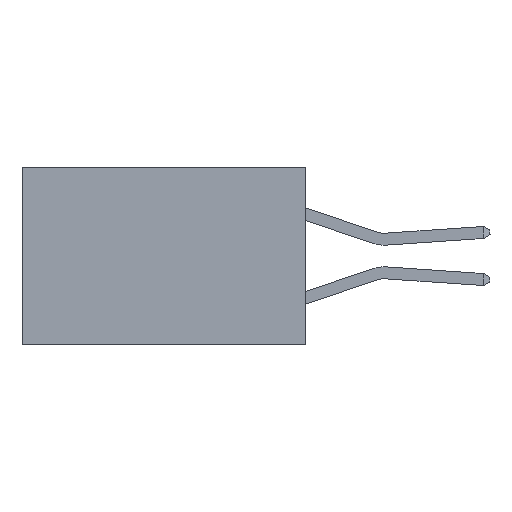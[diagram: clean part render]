
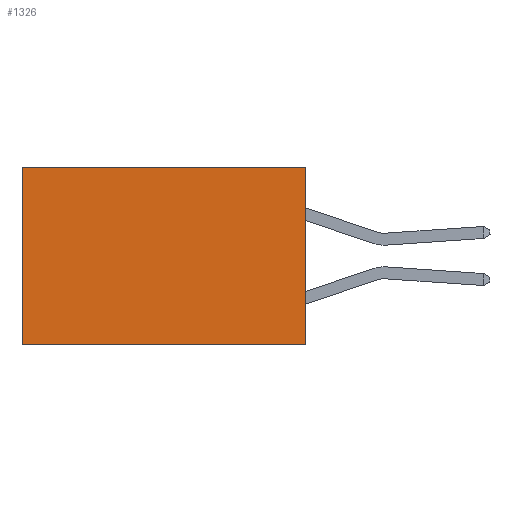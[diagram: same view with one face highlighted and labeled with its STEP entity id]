
A CAD part, left-side view. The second image highlights one B-rep face of the part: STEP entity #1326.
In plain terms, the highlighted planar face has unit normal (-1, 0, 0).
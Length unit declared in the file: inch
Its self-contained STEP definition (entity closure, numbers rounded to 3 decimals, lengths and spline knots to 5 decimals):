
#516 = CARTESIAN_POINT ( 'NONE',  ( 0.277, 0., -0.37 ) ) ;
#844 = ORIENTED_EDGE ( 'NONE', *, *, #13357, .F. ) ;
#1084 = VECTOR ( 'NONE', #12123, 39.37008 ) ;
#1326 = ADVANCED_FACE ( 'NONE', ( #5445 ), #11042, .F. ) ;
#1681 = VERTEX_POINT ( 'NONE', #4177 ) ;
#1693 = LINE ( 'NONE', #2842, #13800 ) ;
#1910 = EDGE_CURVE ( 'NONE', #21023, #1681, #1693, .T. ) ;
#2842 = CARTESIAN_POINT ( 'NONE',  ( 0.277, 0., -0.37 ) ) ;
#3758 = CARTESIAN_POINT ( 'NONE',  ( 0.277, 0., 0. ) ) ;
#3918 = CARTESIAN_POINT ( 'NONE',  ( 0.277, 0., -0.37 ) ) ;
#3971 = EDGE_CURVE ( 'NONE', #13083, #1681, #19894, .T. ) ;
#4177 = CARTESIAN_POINT ( 'NONE',  ( 0.277, 0.59, -0.37 ) ) ;
#4733 = DIRECTION ( 'NONE',  ( 0., 1., 0. ) ) ;
#4992 = ORIENTED_EDGE ( 'NONE', *, *, #1910, .F. ) ;
#5445 = FACE_OUTER_BOUND ( 'NONE', #12772, .T. ) ;
#5502 = DIRECTION ( 'NONE',  ( 0., 1., 0. ) ) ;
#6161 = LINE ( 'NONE', #3918, #1084 ) ;
#6431 = VERTEX_POINT ( 'NONE', #7414 ) ;
#6675 = VECTOR ( 'NONE', #5502, 39.37008 ) ;
#6808 = CARTESIAN_POINT ( 'NONE',  ( 0.277, 0., -0.37 ) ) ;
#7414 = CARTESIAN_POINT ( 'NONE',  ( 0.277, 0., 0. ) ) ;
#7628 = VECTOR ( 'NONE', #14537, 39.37008 ) ;
#8742 = ORIENTED_EDGE ( 'NONE', *, *, #13300, .T. ) ;
#9762 = ORIENTED_EDGE ( 'NONE', *, *, #3971, .T. ) ;
#10897 = DIRECTION ( 'NONE',  ( 1., 0., 0. ) ) ;
#11042 = PLANE ( 'NONE',  #17449 ) ;
#11395 = CARTESIAN_POINT ( 'NONE',  ( 0.277, 0.59, -0.37 ) ) ;
#11501 = LINE ( 'NONE', #3758, #6675 ) ;
#12123 = DIRECTION ( 'NONE',  ( 0., 0., -1. ) ) ;
#12723 = DIRECTION ( 'NONE',  ( 0., 0., -1. ) ) ;
#12772 = EDGE_LOOP ( 'NONE', ( #9762, #4992, #844, #8742 ) ) ;
#13083 = VERTEX_POINT ( 'NONE', #16232 ) ;
#13300 = EDGE_CURVE ( 'NONE', #6431, #13083, #11501, .T. ) ;
#13357 = EDGE_CURVE ( 'NONE', #6431, #21023, #6161, .T. ) ;
#13800 = VECTOR ( 'NONE', #4733, 39.37008 ) ;
#14537 = DIRECTION ( 'NONE',  ( 0., 0., -1. ) ) ;
#16232 = CARTESIAN_POINT ( 'NONE',  ( 0.277, 0.59, 0. ) ) ;
#17449 = AXIS2_PLACEMENT_3D ( 'NONE', #6808, #10897, #12723 ) ;
#19894 = LINE ( 'NONE', #11395, #7628 ) ;
#21023 = VERTEX_POINT ( 'NONE', #516 ) ;
